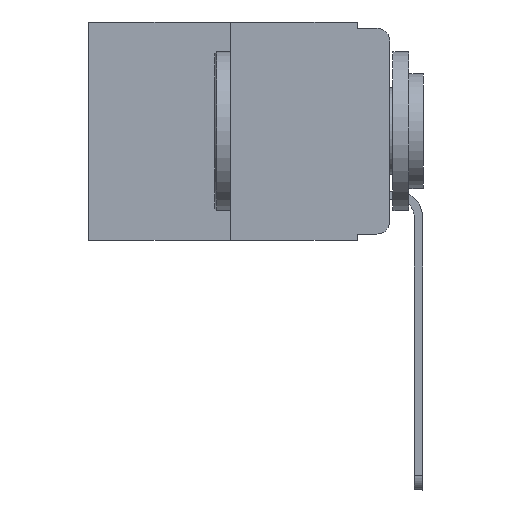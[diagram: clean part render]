
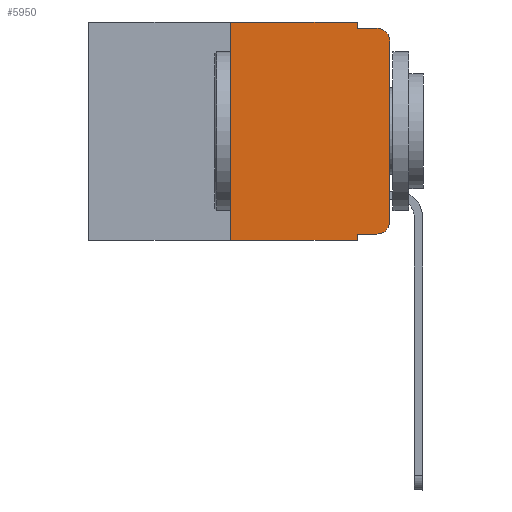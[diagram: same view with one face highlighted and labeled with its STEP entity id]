
A CAD part, left-side view. The second image highlights one B-rep face of the part: STEP entity #5950.
In plain terms, the highlighted planar face has unit normal (-1, 0, 0).
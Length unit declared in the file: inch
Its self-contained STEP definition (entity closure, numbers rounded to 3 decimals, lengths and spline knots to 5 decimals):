
#1043 = CARTESIAN_POINT ( 'NONE',  ( 0., 0., -0.313 ) ) ;
#1116 = DIRECTION ( 'NONE',  ( -1., 0., 0. ) ) ;
#1213 = LINE ( 'NONE', #17696, #15512 ) ;
#1871 = CARTESIAN_POINT ( 'NONE',  ( 0., 0., -0.03 ) ) ;
#2571 = CARTESIAN_POINT ( 'NONE',  ( 0., 0., 0. ) ) ;
#2916 = LINE ( 'NONE', #25798, #6979 ) ;
#2989 = CARTESIAN_POINT ( 'NONE',  ( 0., 0.473, 0. ) ) ;
#3053 = CARTESIAN_POINT ( 'NONE',  ( 0., 0.473, -0.343 ) ) ;
#3076 = CARTESIAN_POINT ( 'NONE',  ( 0., 0.25, 0. ) ) ;
#3345 = EDGE_CURVE ( 'NONE', #12143, #15905, #2916, .T. ) ;
#3491 = EDGE_CURVE ( 'NONE', #13069, #6843, #18422, .T. ) ;
#3686 = CARTESIAN_POINT ( 'NONE',  ( 0., 0.051, -0.01 ) ) ;
#3717 = CARTESIAN_POINT ( 'NONE',  ( 0., 0.473, 0. ) ) ;
#4155 = EDGE_CURVE ( 'NONE', #20837, #20659, #23823, .T. ) ;
#4851 = VECTOR ( 'NONE', #23636, 39.37008 ) ;
#5011 = DIRECTION ( 'NONE',  ( 0., 0., 1. ) ) ;
#5124 = EDGE_CURVE ( 'NONE', #17473, #14883, #9302, .T. ) ;
#5277 = DIRECTION ( 'NONE',  ( 0., -1., 0. ) ) ;
#5524 = AXIS2_PLACEMENT_3D ( 'NONE', #22455, #1116, #25911 ) ;
#5911 = AXIS2_PLACEMENT_3D ( 'NONE', #7329, #9501, #21905 ) ;
#5950 = ADVANCED_FACE ( 'NONE', ( #13330 ), #19995, .F. ) ;
#6601 = ORIENTED_EDGE ( 'NONE', *, *, #8419, .F. ) ;
#6843 = VERTEX_POINT ( 'NONE', #7498 ) ;
#6979 = VECTOR ( 'NONE', #7118, 39.37008 ) ;
#7011 = CARTESIAN_POINT ( 'NONE',  ( 0., 0.051, 0. ) ) ;
#7118 = DIRECTION ( 'NONE',  ( 0., -1., 0. ) ) ;
#7293 = DIRECTION ( 'NONE',  ( 0., 0., 1. ) ) ;
#7329 = CARTESIAN_POINT ( 'NONE',  ( 0., 0.02, -0.313 ) ) ;
#7384 = CARTESIAN_POINT ( 'NONE',  ( 0., 0.051, -0.343 ) ) ;
#7498 = CARTESIAN_POINT ( 'NONE',  ( 0., 0.051, 0. ) ) ;
#8051 = DIRECTION ( 'NONE',  ( 0., -1., 0. ) ) ;
#8065 = CARTESIAN_POINT ( 'NONE',  ( 0., 0.051, -0.333 ) ) ;
#8419 = EDGE_CURVE ( 'NONE', #6843, #12143, #21366, .T. ) ;
#8558 = CARTESIAN_POINT ( 'NONE',  ( 0., 0.051, 0. ) ) ;
#8654 = VECTOR ( 'NONE', #18033, 39.37008 ) ;
#9302 = LINE ( 'NONE', #3053, #8654 ) ;
#9501 = DIRECTION ( 'NONE',  ( -1., 0., 0. ) ) ;
#10187 = VECTOR ( 'NONE', #7293, 39.37008 ) ;
#10891 = VECTOR ( 'NONE', #8051, 39.37008 ) ;
#11541 = CIRCLE ( 'NONE', #5911, 0.02 ) ;
#12143 = VERTEX_POINT ( 'NONE', #3686 ) ;
#12197 = CARTESIAN_POINT ( 'NONE',  ( 0., 0.25, 0. ) ) ;
#12476 = EDGE_CURVE ( 'NONE', #24114, #21746, #1213, .T. ) ;
#13069 = VERTEX_POINT ( 'NONE', #12197 ) ;
#13330 = FACE_OUTER_BOUND ( 'NONE', #23463, .T. ) ;
#13409 = ORIENTED_EDGE ( 'NONE', *, *, #20878, .F. ) ;
#13454 = ORIENTED_EDGE ( 'NONE', *, *, #24971, .T. ) ;
#14500 = ORIENTED_EDGE ( 'NONE', *, *, #19003, .F. ) ;
#14883 = VERTEX_POINT ( 'NONE', #7384 ) ;
#14924 = ORIENTED_EDGE ( 'NONE', *, *, #23656, .T. ) ;
#15022 = ORIENTED_EDGE ( 'NONE', *, *, #5124, .T. ) ;
#15512 = VECTOR ( 'NONE', #5277, 39.37008 ) ;
#15905 = VERTEX_POINT ( 'NONE', #16045 ) ;
#15912 = AXIS2_PLACEMENT_3D ( 'NONE', #2989, #21763, #17698 ) ;
#16045 = CARTESIAN_POINT ( 'NONE',  ( 0., 0.02, -0.01 ) ) ;
#16821 = CIRCLE ( 'NONE', #5524, 0.02 ) ;
#17473 = VERTEX_POINT ( 'NONE', #20778 ) ;
#17696 = CARTESIAN_POINT ( 'NONE',  ( 0., 0.051, -0.333 ) ) ;
#17698 = DIRECTION ( 'NONE',  ( 0., 0., -1. ) ) ;
#18033 = DIRECTION ( 'NONE',  ( 0., -1., 0. ) ) ;
#18397 = ORIENTED_EDGE ( 'NONE', *, *, #12476, .T. ) ;
#18422 = LINE ( 'NONE', #3717, #10891 ) ;
#18647 = ORIENTED_EDGE ( 'NONE', *, *, #4155, .T. ) ;
#19003 = EDGE_CURVE ( 'NONE', #24114, #14883, #25683, .T. ) ;
#19211 = ORIENTED_EDGE ( 'NONE', *, *, #3345, .F. ) ;
#19995 = PLANE ( 'NONE',  #15912 ) ;
#20659 = VERTEX_POINT ( 'NONE', #1871 ) ;
#20724 = VECTOR ( 'NONE', #21096, 39.37008 ) ;
#20778 = CARTESIAN_POINT ( 'NONE',  ( 0., 0.25, -0.343 ) ) ;
#20837 = VERTEX_POINT ( 'NONE', #1043 ) ;
#20878 = EDGE_CURVE ( 'NONE', #17473, #13069, #23508, .T. ) ;
#21096 = DIRECTION ( 'NONE',  ( 0., 0., -1. ) ) ;
#21366 = LINE ( 'NONE', #8558, #20724 ) ;
#21746 = VERTEX_POINT ( 'NONE', #23036 ) ;
#21763 = DIRECTION ( 'NONE',  ( 1., 0., 0. ) ) ;
#21905 = DIRECTION ( 'NONE',  ( 0., 0., -1. ) ) ;
#22257 = VECTOR ( 'NONE', #5011, 39.37008 ) ;
#22455 = CARTESIAN_POINT ( 'NONE',  ( 0., 0.02, -0.03 ) ) ;
#22674 = ORIENTED_EDGE ( 'NONE', *, *, #3491, .F. ) ;
#23036 = CARTESIAN_POINT ( 'NONE',  ( 0., 0.02, -0.333 ) ) ;
#23463 = EDGE_LOOP ( 'NONE', ( #18647, #13454, #19211, #6601, #22674, #13409, #15022, #14500, #18397, #14924 ) ) ;
#23508 = LINE ( 'NONE', #3076, #10187 ) ;
#23636 = DIRECTION ( 'NONE',  ( 0., 0., -1. ) ) ;
#23656 = EDGE_CURVE ( 'NONE', #21746, #20837, #11541, .T. ) ;
#23823 = LINE ( 'NONE', #2571, #22257 ) ;
#24114 = VERTEX_POINT ( 'NONE', #8065 ) ;
#24971 = EDGE_CURVE ( 'NONE', #20659, #15905, #16821, .T. ) ;
#25683 = LINE ( 'NONE', #7011, #4851 ) ;
#25798 = CARTESIAN_POINT ( 'NONE',  ( 0., 0.051, -0.01 ) ) ;
#25911 = DIRECTION ( 'NONE',  ( 0., 0., -1. ) ) ;
